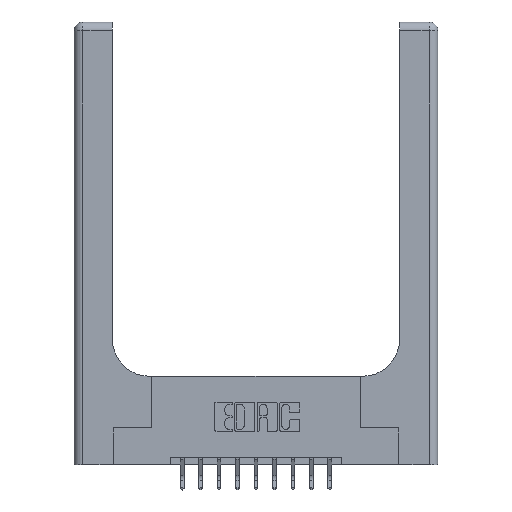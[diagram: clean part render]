
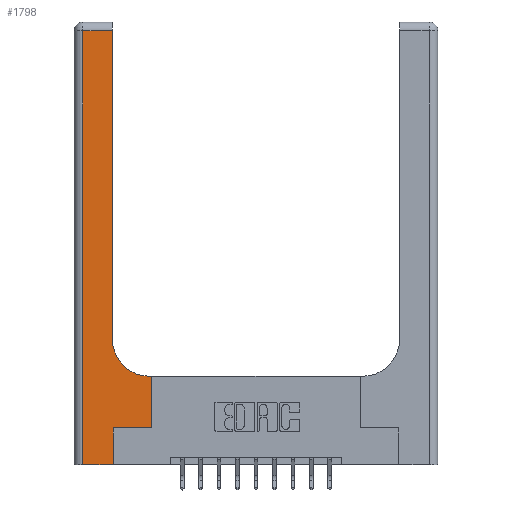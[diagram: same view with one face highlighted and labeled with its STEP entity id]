
A CAD part, top view. The second image highlights one B-rep face of the part: STEP entity #1798.
In plain terms, the highlighted planar face has unit normal (0, 0, 1).
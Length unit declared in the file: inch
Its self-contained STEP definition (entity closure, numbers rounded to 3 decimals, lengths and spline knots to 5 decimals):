
#55 = CARTESIAN_POINT ( 'NONE',  ( 0.51, 0.6, 0.37 ) ) ;
#113 = VERTEX_POINT ( 'NONE', #3300 ) ;
#202 = CIRCLE ( 'NONE', #7702, 0.25 ) ;
#1243 = CARTESIAN_POINT ( 'NONE',  ( 0.51, 0.85, 0.37 ) ) ;
#1717 = ORIENTED_EDGE ( 'NONE', *, *, #15016, .T. ) ;
#1798 = ADVANCED_FACE ( 'NONE', ( #11021 ), #11783, .F. ) ;
#1891 = EDGE_CURVE ( 'NONE', #7897, #113, #14668, .T. ) ;
#2126 = EDGE_LOOP ( 'NONE', ( #3776, #6156, #8850, #14699, #15096, #4643, #1717, #7144, #11884 ) ) ;
#2411 = VERTEX_POINT ( 'NONE', #12911 ) ;
#2544 = LINE ( 'NONE', #13876, #5366 ) ;
#2579 = CARTESIAN_POINT ( 'NONE',  ( 0.528, 0.25, 0.37 ) ) ;
#2960 = VECTOR ( 'NONE', #5505, 39.37008 ) ;
#3062 = EDGE_CURVE ( 'NONE', #10184, #13046, #14636, .T. ) ;
#3300 = CARTESIAN_POINT ( 'NONE',  ( 0.26, 2.94, 0.37 ) ) ;
#3473 = VERTEX_POINT ( 'NONE', #4159 ) ;
#3776 = ORIENTED_EDGE ( 'NONE', *, *, #1891, .T. ) ;
#4159 = CARTESIAN_POINT ( 'NONE',  ( 0.528, 0.25, 0.37 ) ) ;
#4176 = DIRECTION ( 'NONE',  ( -1., 0., 0. ) ) ;
#4278 = LINE ( 'NONE', #13815, #13203 ) ;
#4643 = ORIENTED_EDGE ( 'NONE', *, *, #6619, .T. ) ;
#5366 = VECTOR ( 'NONE', #4176, 39.37008 ) ;
#5505 = DIRECTION ( 'NONE',  ( 0., -1., 0. ) ) ;
#5861 = VERTEX_POINT ( 'NONE', #15394 ) ;
#6156 = ORIENTED_EDGE ( 'NONE', *, *, #9061, .T. ) ;
#6222 = DIRECTION ( 'NONE',  ( 1., 0., 0. ) ) ;
#6330 = DIRECTION ( 'NONE',  ( 1., 0., 0. ) ) ;
#6619 = EDGE_CURVE ( 'NONE', #5861, #3473, #8633, .T. ) ;
#6647 = DIRECTION ( 'NONE',  ( 0., 0., -1. ) ) ;
#6699 = DIRECTION ( 'NONE',  ( -1., 0., 0. ) ) ;
#6835 = CARTESIAN_POINT ( 'NONE',  ( 0.26, 3., 0.37 ) ) ;
#7036 = CARTESIAN_POINT ( 'NONE',  ( 0., 3., 0.37 ) ) ;
#7144 = ORIENTED_EDGE ( 'NONE', *, *, #3062, .T. ) ;
#7249 = VECTOR ( 'NONE', #11742, 39.37008 ) ;
#7702 = AXIS2_PLACEMENT_3D ( 'NONE', #1243, #13484, #9702 ) ;
#7897 = VERTEX_POINT ( 'NONE', #8684 ) ;
#8021 = VERTEX_POINT ( 'NONE', #13981 ) ;
#8358 = EDGE_CURVE ( 'NONE', #8021, #2411, #12226, .T. ) ;
#8630 = EDGE_CURVE ( 'NONE', #2411, #5861, #4278, .T. ) ;
#8633 = LINE ( 'NONE', #9877, #12857 ) ;
#8684 = CARTESIAN_POINT ( 'NONE',  ( 0.26, 0.85, 0.37 ) ) ;
#8850 = ORIENTED_EDGE ( 'NONE', *, *, #12187, .T. ) ;
#8983 = VECTOR ( 'NONE', #6222, 39.37008 ) ;
#9061 = EDGE_CURVE ( 'NONE', #113, #9746, #2544, .T. ) ;
#9513 = DIRECTION ( 'NONE',  ( -1., 0., 0. ) ) ;
#9702 = DIRECTION ( 'NONE',  ( 1., 0., 0. ) ) ;
#9746 = VERTEX_POINT ( 'NONE', #11498 ) ;
#9877 = CARTESIAN_POINT ( 'NONE',  ( 0.265, 0.25, 0.37 ) ) ;
#9928 = LINE ( 'NONE', #2579, #12197 ) ;
#10184 = VERTEX_POINT ( 'NONE', #14984 ) ;
#10457 = EDGE_CURVE ( 'NONE', #13046, #7897, #202, .T. ) ;
#10597 = VECTOR ( 'NONE', #9513, 39.37008 ) ;
#11021 = FACE_OUTER_BOUND ( 'NONE', #2126, .T. ) ;
#11066 = AXIS2_PLACEMENT_3D ( 'NONE', #7036, #6647, #6699 ) ;
#11078 = DIRECTION ( 'NONE',  ( 0., 1., 0. ) ) ;
#11498 = CARTESIAN_POINT ( 'NONE',  ( 0.06, 2.94, 0.37 ) ) ;
#11742 = DIRECTION ( 'NONE',  ( 0., 1., 0. ) ) ;
#11783 = PLANE ( 'NONE',  #11066 ) ;
#11871 = LINE ( 'NONE', #12773, #2960 ) ;
#11884 = ORIENTED_EDGE ( 'NONE', *, *, #10457, .T. ) ;
#12187 = EDGE_CURVE ( 'NONE', #9746, #8021, #11871, .T. ) ;
#12197 = VECTOR ( 'NONE', #11078, 39.37008 ) ;
#12226 = LINE ( 'NONE', #14729, #8983 ) ;
#12773 = CARTESIAN_POINT ( 'NONE',  ( 0.06, 3., 0.37 ) ) ;
#12857 = VECTOR ( 'NONE', #6330, 39.37008 ) ;
#12911 = CARTESIAN_POINT ( 'NONE',  ( 0.265, 0., 0.37 ) ) ;
#13046 = VERTEX_POINT ( 'NONE', #55 ) ;
#13203 = VECTOR ( 'NONE', #15427, 39.37008 ) ;
#13484 = DIRECTION ( 'NONE',  ( 0., 0., -1. ) ) ;
#13815 = CARTESIAN_POINT ( 'NONE',  ( 0.265, 0., 0.37 ) ) ;
#13876 = CARTESIAN_POINT ( 'NONE',  ( 0., 2.94, 0.37 ) ) ;
#13981 = CARTESIAN_POINT ( 'NONE',  ( 0.06, 0., 0.37 ) ) ;
#14636 = LINE ( 'NONE', #15612, #10597 ) ;
#14668 = LINE ( 'NONE', #6835, #7249 ) ;
#14699 = ORIENTED_EDGE ( 'NONE', *, *, #8358, .T. ) ;
#14729 = CARTESIAN_POINT ( 'NONE',  ( 0., 0., 0.37 ) ) ;
#14984 = CARTESIAN_POINT ( 'NONE',  ( 0.528, 0.6, 0.37 ) ) ;
#15016 = EDGE_CURVE ( 'NONE', #3473, #10184, #9928, .T. ) ;
#15096 = ORIENTED_EDGE ( 'NONE', *, *, #8630, .T. ) ;
#15394 = CARTESIAN_POINT ( 'NONE',  ( 0.265, 0.25, 0.37 ) ) ;
#15427 = DIRECTION ( 'NONE',  ( 0., 1., 0. ) ) ;
#15612 = CARTESIAN_POINT ( 'NONE',  ( 0.26, 0.6, 0.37 ) ) ;
